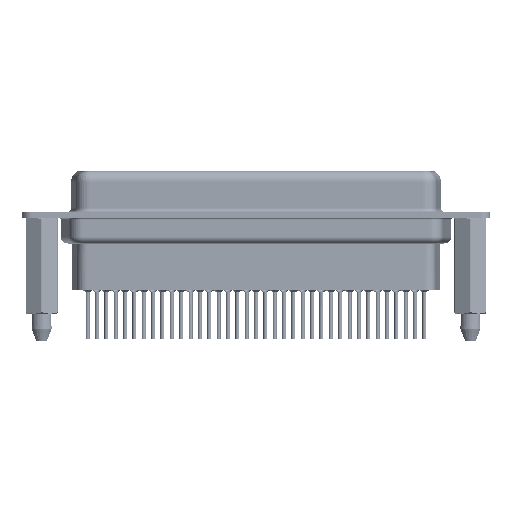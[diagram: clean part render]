
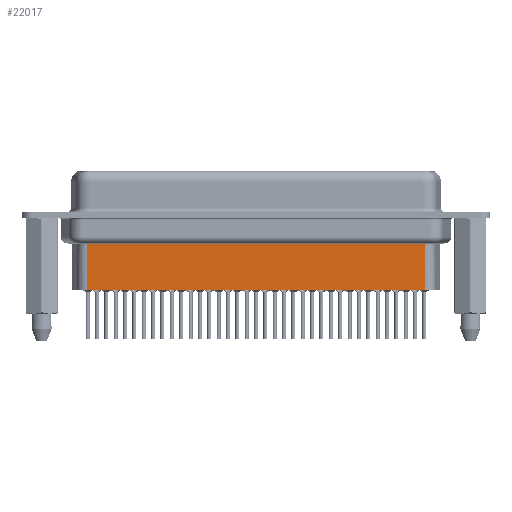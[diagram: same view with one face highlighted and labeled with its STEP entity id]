
A CAD part, front view. The second image highlights one B-rep face of the part: STEP entity #22017.
In plain terms, the highlighted planar face has unit normal (0, -1, 0).
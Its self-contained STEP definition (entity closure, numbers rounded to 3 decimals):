
#2006 = EDGE_CURVE ( 'NONE', #21349, #3548, #28832, .T. ) ;
#2996 = CARTESIAN_POINT ( 'NONE',  ( 6.706, -3.5, -4.097 ) ) ;
#3207 = CARTESIAN_POINT ( 'NONE',  ( 56.794, -3.5, -11.15 ) ) ;
#3548 = VERTEX_POINT ( 'NONE', #20974 ) ;
#6285 = CARTESIAN_POINT ( 'NONE',  ( 56.794, -3.5, -3.1 ) ) ;
#6614 = DIRECTION ( 'NONE',  ( 0., 0., -1. ) ) ;
#7621 = EDGE_LOOP ( 'NONE', ( #17253, #32007, #13744, #19287 ) ) ;
#8497 = EDGE_CURVE ( 'NONE', #25298, #3548, #21849, .T. ) ;
#9907 = EDGE_CURVE ( 'NONE', #18600, #25298, #30693, .T. ) ;
#10321 = FACE_OUTER_BOUND ( 'NONE', #7621, .T. ) ;
#12201 = CARTESIAN_POINT ( 'NONE',  ( 6.706, -3.5, -3.1 ) ) ;
#13744 = ORIENTED_EDGE ( 'NONE', *, *, #8497, .T. ) ;
#15759 = CARTESIAN_POINT ( 'NONE',  ( 56.794, -3.5, -4.097 ) ) ;
#17253 = ORIENTED_EDGE ( 'NONE', *, *, #32983, .F. ) ;
#18044 = DIRECTION ( 'NONE',  ( 0., -1., 0. ) ) ;
#18600 = VERTEX_POINT ( 'NONE', #15759 ) ;
#19100 = CARTESIAN_POINT ( 'NONE',  ( 6.706, -3.5, -3.1 ) ) ;
#19273 = DIRECTION ( 'NONE',  ( 0., 0., -1. ) ) ;
#19287 = ORIENTED_EDGE ( 'NONE', *, *, #2006, .F. ) ;
#20095 = AXIS2_PLACEMENT_3D ( 'NONE', #12201, #18044, #20807 ) ;
#20763 = VECTOR ( 'NONE', #6614, 1000. ) ;
#20807 = DIRECTION ( 'NONE',  ( 1., 0., 0. ) ) ;
#20815 = VECTOR ( 'NONE', #22836, 1000. ) ;
#20974 = CARTESIAN_POINT ( 'NONE',  ( 6.706, -3.5, -11.15 ) ) ;
#21349 = VERTEX_POINT ( 'NONE', #3207 ) ;
#21595 = VECTOR ( 'NONE', #24043, 1000. ) ;
#21849 = LINE ( 'NONE', #19100, #23922 ) ;
#22017 = ADVANCED_FACE ( 'NONE', ( #10321 ), #30876, .T. ) ;
#22836 = DIRECTION ( 'NONE',  ( -1., 0., 0. ) ) ;
#23922 = VECTOR ( 'NONE', #19273, 1000. ) ;
#24043 = DIRECTION ( 'NONE',  ( -1., 0., 0. ) ) ;
#25298 = VERTEX_POINT ( 'NONE', #2996 ) ;
#28151 = CARTESIAN_POINT ( 'NONE',  ( 6.459, -3.5, -4.097 ) ) ;
#28832 = LINE ( 'NONE', #29180, #21595 ) ;
#29180 = CARTESIAN_POINT ( 'NONE',  ( 6.706, -3.5, -11.15 ) ) ;
#29914 = LINE ( 'NONE', #6285, #20763 ) ;
#30693 = LINE ( 'NONE', #28151, #20815 ) ;
#30876 = PLANE ( 'NONE',  #20095 ) ;
#32007 = ORIENTED_EDGE ( 'NONE', *, *, #9907, .T. ) ;
#32983 = EDGE_CURVE ( 'NONE', #18600, #21349, #29914, .T. ) ;
